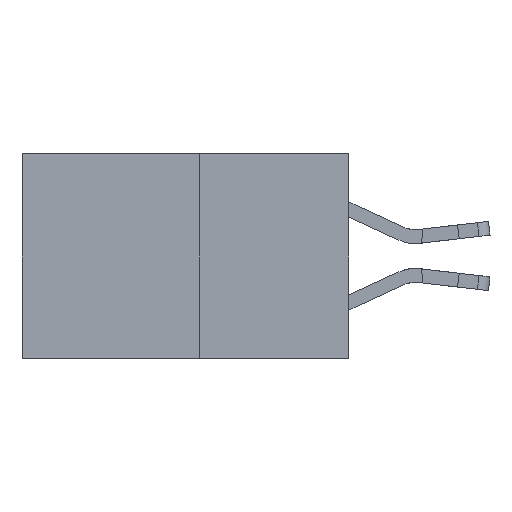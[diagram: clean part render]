
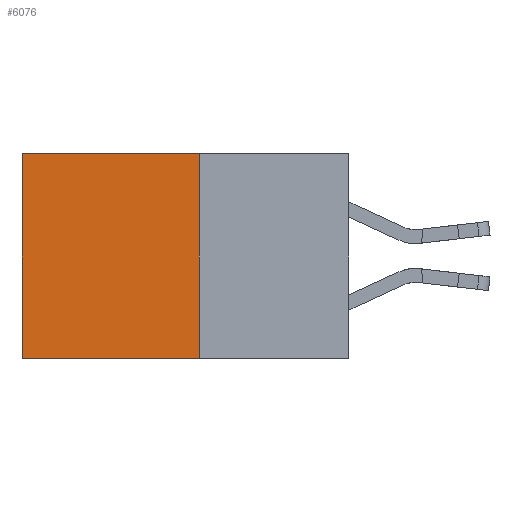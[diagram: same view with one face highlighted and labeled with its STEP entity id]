
A CAD part, left-side view. The second image highlights one B-rep face of the part: STEP entity #6076.
In plain terms, the highlighted planar face has unit normal (-1, 0, 0).
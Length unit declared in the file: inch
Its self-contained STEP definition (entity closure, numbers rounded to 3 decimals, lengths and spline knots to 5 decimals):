
#373 = AXIS2_PLACEMENT_3D ( 'NONE', #12757, #12729, #12702 ) ;
#393 = DIRECTION ( 'NONE',  ( 0., 0., -1. ) ) ;
#1197 = DIRECTION ( 'NONE',  ( 0., 1., 0. ) ) ;
#2995 = CARTESIAN_POINT ( 'NONE',  ( 0.277, 0.27, -0.37 ) ) ;
#2997 = VECTOR ( 'NONE', #11956, 39.37008 ) ;
#4305 = LINE ( 'NONE', #14510, #4828 ) ;
#4828 = VECTOR ( 'NONE', #14330, 39.37008 ) ;
#5056 = CARTESIAN_POINT ( 'NONE',  ( 0.277, 0.59, 0. ) ) ;
#5450 = ORIENTED_EDGE ( 'NONE', *, *, #16753, .F. ) ;
#6076 = ADVANCED_FACE ( 'NONE', ( #7160 ), #12784, .F. ) ;
#7160 = FACE_OUTER_BOUND ( 'NONE', #12146, .T. ) ;
#7166 = VERTEX_POINT ( 'NONE', #19353 ) ;
#7182 = VECTOR ( 'NONE', #1197, 39.37008 ) ;
#7286 = EDGE_CURVE ( 'NONE', #12583, #7166, #4305, .T. ) ;
#9998 = ORIENTED_EDGE ( 'NONE', *, *, #16427, .F. ) ;
#11241 = VERTEX_POINT ( 'NONE', #2995 ) ;
#11956 = DIRECTION ( 'NONE',  ( 0., 1., 0. ) ) ;
#12146 = EDGE_LOOP ( 'NONE', ( #16932, #5450, #9998, #15336 ) ) ;
#12583 = VERTEX_POINT ( 'NONE', #5056 ) ;
#12702 = DIRECTION ( 'NONE',  ( 0., 0., -1. ) ) ;
#12729 = DIRECTION ( 'NONE',  ( 1., 0., 0. ) ) ;
#12757 = CARTESIAN_POINT ( 'NONE',  ( 0.277, 0.27, -0.37 ) ) ;
#12784 = PLANE ( 'NONE',  #373 ) ;
#12811 = VERTEX_POINT ( 'NONE', #18943 ) ;
#14330 = DIRECTION ( 'NONE',  ( 0., 0., -1. ) ) ;
#14510 = CARTESIAN_POINT ( 'NONE',  ( 0.277, 0.59, -0.37 ) ) ;
#15336 = ORIENTED_EDGE ( 'NONE', *, *, #15646, .T. ) ;
#15646 = EDGE_CURVE ( 'NONE', #12811, #12583, #20817, .T. ) ;
#16085 = LINE ( 'NONE', #21283, #7182 ) ;
#16427 = EDGE_CURVE ( 'NONE', #12811, #11241, #18448, .T. ) ;
#16753 = EDGE_CURVE ( 'NONE', #11241, #7166, #16085, .T. ) ;
#16932 = ORIENTED_EDGE ( 'NONE', *, *, #7286, .T. ) ;
#17908 = VECTOR ( 'NONE', #393, 39.37008 ) ;
#18448 = LINE ( 'NONE', #18844, #17908 ) ;
#18844 = CARTESIAN_POINT ( 'NONE',  ( 0.277, 0.27, -0.37 ) ) ;
#18943 = CARTESIAN_POINT ( 'NONE',  ( 0.277, 0.27, 0. ) ) ;
#19353 = CARTESIAN_POINT ( 'NONE',  ( 0.277, 0.59, -0.37 ) ) ;
#20256 = CARTESIAN_POINT ( 'NONE',  ( 0.277, 0.27, 0. ) ) ;
#20817 = LINE ( 'NONE', #20256, #2997 ) ;
#21283 = CARTESIAN_POINT ( 'NONE',  ( 0.277, 0.27, -0.37 ) ) ;
